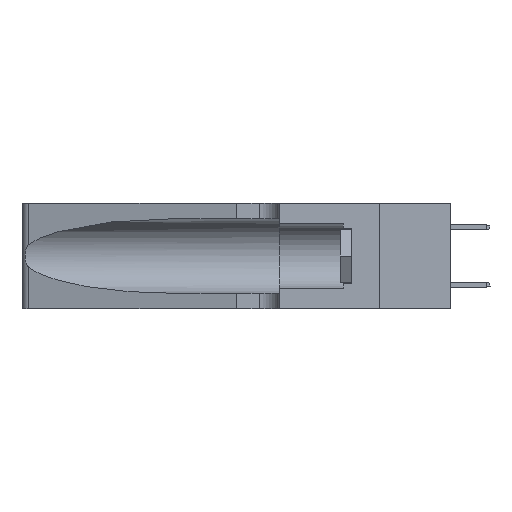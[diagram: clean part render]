
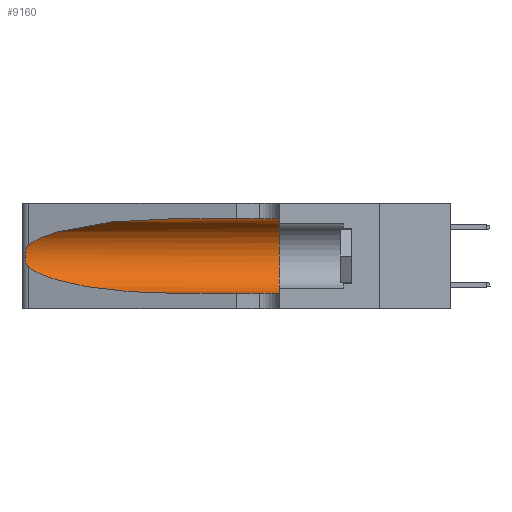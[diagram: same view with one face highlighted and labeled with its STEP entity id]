
A CAD part, left-side view. The second image highlights one B-rep face of the part: STEP entity #9160.
In plain terms, the highlighted cylindrical face has radius 3.308 mm (diameter 6.617 mm), a partial arc.
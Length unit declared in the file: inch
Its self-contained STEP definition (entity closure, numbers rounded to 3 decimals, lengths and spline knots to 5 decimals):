
#582 = EDGE_CURVE ( 'NONE', #22631, #23381, #16687, .T. ) ;
#751 = CARTESIAN_POINT ( 'NONE',  ( 0.25487, 1.22718, 0.14631 ) ) ;
#968 = CARTESIAN_POINT ( 'NONE',  ( 0.25487, 1.22718, 0.22369 ) ) ;
#1366 = ORIENTED_EDGE ( 'NONE', *, *, #582, .T. ) ;
#1863 = DIRECTION ( 'NONE',  ( 0., -1., 0. ) ) ;
#1893 = CARTESIAN_POINT ( 'NONE',  ( 0.26075, 1.23896, 0.19203 ) ) ;
#2206 = CARTESIAN_POINT ( 'NONE',  ( 0.25487, 1.22718, 0.22369 ) ) ;
#3266 = ORIENTED_EDGE ( 'NONE', *, *, #9719, .T. ) ;
#3587 = FACE_OUTER_BOUND ( 'NONE', #12122, .T. ) ;
#3680 = CARTESIAN_POINT ( 'NONE',  ( 0.2373, 1.15595, 0.08982 ) ) ;
#3694 = CARTESIAN_POINT ( 'NONE',  ( 0.25487, 1.22718, 0.22369 ) ) ;
#3941 = LINE ( 'NONE', #12387, #14306 ) ;
#4221 = ORIENTED_EDGE ( 'NONE', *, *, #21253, .F. ) ;
#5030 = ORIENTED_EDGE ( 'NONE', *, *, #7592, .T. ) ;
#6502 = CARTESIAN_POINT ( 'NONE',  ( 0.18966, 0.96281, 0.31525 ) ) ;
#6540 = EDGE_CURVE ( 'NONE', #23381, #25996, #3941, .T. ) ;
#7072 = CARTESIAN_POINT ( 'NONE',  ( 0.1305, 1.61858, 0.31525 ) ) ;
#7592 = EDGE_CURVE ( 'NONE', #16928, #26767, #19311, .T. ) ;
#7819 = CARTESIAN_POINT ( 'NONE',  ( 0.25487, 1.22718, 0.14631 ) ) ;
#7873 = CYLINDRICAL_SURFACE ( 'NONE', #8677, 0.13025 ) ;
#8677 = AXIS2_PLACEMENT_3D ( 'NONE', #16222, #23913, #21814 ) ;
#8712 = VECTOR ( 'NONE', #25985, 39.37008 ) ;
#9160 = ADVANCED_FACE ( 'NONE', ( #3587 ), #7873, .F. ) ;
#9719 = EDGE_CURVE ( 'NONE', #26767, #22631, #20404, .T. ) ;
#11981 = CARTESIAN_POINT ( 'NONE',  ( 0.18966, 0.96281, 0.05475 ) ) ;
#12122 = EDGE_LOOP ( 'NONE', ( #5030, #3266, #1366, #23054, #4221, #24940 ) ) ;
#12138 = CARTESIAN_POINT ( 'NONE',  ( 0.26018, 1.23835, 0.19895 ) ) ;
#12283 = CARTESIAN_POINT ( 'NONE',  ( 0.25487, 1.22718, 0.14631 ) ) ;
#12387 = CARTESIAN_POINT ( 'NONE',  ( 0.1305, 1.61858, 0.05475 ) ) ;
#12556 = CARTESIAN_POINT ( 'NONE',  ( 0.26075, 1.23896, 0.178 ) ) ;
#12794 = DIRECTION ( 'NONE',  ( 0., 0., 1. ) ) ;
#13664 = CARTESIAN_POINT ( 'NONE',  ( 0.1305, 0.72297, 0.05475 ) ) ;
#14236 = CARTESIAN_POINT ( 'NONE',  ( 0.25854, 1.2359, 0.20912 ) ) ;
#14306 = VECTOR ( 'NONE', #1863, 39.37008 ) ;
#14658 = CARTESIAN_POINT ( 'NONE',  ( 0.25555, 1.22994, 0.2215 ) ) ;
#14836 = VERTEX_POINT ( 'NONE', #26841 ) ;
#15714 = CARTESIAN_POINT ( 'NONE',  ( 0.25555, 1.22993, 0.14849 ) ) ;
#16146 = CARTESIAN_POINT ( 'NONE',  ( 0.1305, 0.35, 0.05475 ) ) ;
#16222 = CARTESIAN_POINT ( 'NONE',  ( 0.1305, 1.61858, 0.185 ) ) ;
#16470 = CARTESIAN_POINT ( 'NONE',  ( 0.25787, 1.23484, 0.2124 ) ) ;
#16687 =( BOUNDED_CURVE ( )  B_SPLINE_CURVE ( 3, ( #7819, #3680, #11981, #13664 ),
 .UNSPECIFIED., .F., .F. ) 
 B_SPLINE_CURVE_WITH_KNOTS ( ( 4, 4 ),
 ( 3.44316, 4.71239 ),
 .UNSPECIFIED. ) 
 CURVE ( )  GEOMETRIC_REPRESENTATION_ITEM ( )  RATIONAL_B_SPLINE_CURVE ( ( 1., 0.87, 0.87, 1. ) ) 
 REPRESENTATION_ITEM ( '' )  );
#16777 = CIRCLE ( 'NONE', #21652, 0.13025 ) ;
#16911 = CARTESIAN_POINT ( 'NONE',  ( 0.2373, 1.15595, 0.28018 ) ) ;
#16928 = VERTEX_POINT ( 'NONE', #17889 ) ;
#16967 = CARTESIAN_POINT ( 'NONE',  ( 0.1305, 0.35, 0.185 ) ) ;
#17179 = CARTESIAN_POINT ( 'NONE',  ( 0.1305, 0.72297, 0.31525 ) ) ;
#17889 = CARTESIAN_POINT ( 'NONE',  ( 0.1305, 0.72297, 0.31525 ) ) ;
#18551 = CARTESIAN_POINT ( 'NONE',  ( 0.25639, 1.23186, 0.15144 ) ) ;
#19311 =( BOUNDED_CURVE ( )  B_SPLINE_CURVE ( 3, ( #17179, #6502, #16911, #2206 ),
 .UNSPECIFIED., .F., .F. ) 
 B_SPLINE_CURVE_WITH_KNOTS ( ( 4, 4 ),
 ( 1.5708, 2.84003 ),
 .UNSPECIFIED. ) 
 CURVE ( )  GEOMETRIC_REPRESENTATION_ITEM ( )  RATIONAL_B_SPLINE_CURVE ( ( 1., 0.87, 0.87, 1. ) ) 
 REPRESENTATION_ITEM ( '' )  );
#20028 = EDGE_CURVE ( 'NONE', #16928, #14836, #25702, .T. ) ;
#20404 = B_SPLINE_CURVE_WITH_KNOTS ( 'NONE', 3,
 ( #3694, #14658, #25356, #16470, #14236, #12138, #1893, #12556, #22709, #24801, #20632, #18551, #15714, #12283 ),
 .UNSPECIFIED., .F., .F.,
 ( 4, 2, 2, 2, 2, 2, 4 ),
 ( 0., 0.00027, 0.00053, 0.00107, 0.0016, 0.00187, 0.00214 ),
 .UNSPECIFIED. ) ;
#20632 = CARTESIAN_POINT ( 'NONE',  ( 0.25789, 1.23486, 0.15765 ) ) ;
#21253 = EDGE_CURVE ( 'NONE', #14836, #25996, #16777, .T. ) ;
#21652 = AXIS2_PLACEMENT_3D ( 'NONE', #16967, #23232, #12794 ) ;
#21814 = DIRECTION ( 'NONE',  ( 0., 0., -1. ) ) ;
#22631 = VERTEX_POINT ( 'NONE', #751 ) ;
#22709 = CARTESIAN_POINT ( 'NONE',  ( 0.26017, 1.23833, 0.17102 ) ) ;
#22899 = CARTESIAN_POINT ( 'NONE',  ( 0.1305, 0.72297, 0.05475 ) ) ;
#23054 = ORIENTED_EDGE ( 'NONE', *, *, #6540, .T. ) ;
#23232 = DIRECTION ( 'NONE',  ( 0., 1., 0. ) ) ;
#23381 = VERTEX_POINT ( 'NONE', #22899 ) ;
#23913 = DIRECTION ( 'NONE',  ( 0., -1., 0. ) ) ;
#24801 = CARTESIAN_POINT ( 'NONE',  ( 0.25856, 1.23593, 0.16098 ) ) ;
#24940 = ORIENTED_EDGE ( 'NONE', *, *, #20028, .F. ) ;
#25356 = CARTESIAN_POINT ( 'NONE',  ( 0.25639, 1.23184, 0.21858 ) ) ;
#25702 = LINE ( 'NONE', #7072, #8712 ) ;
#25985 = DIRECTION ( 'NONE',  ( 0., -1., 0. ) ) ;
#25996 = VERTEX_POINT ( 'NONE', #16146 ) ;
#26767 = VERTEX_POINT ( 'NONE', #968 ) ;
#26841 = CARTESIAN_POINT ( 'NONE',  ( 0.1305, 0.35, 0.31525 ) ) ;
